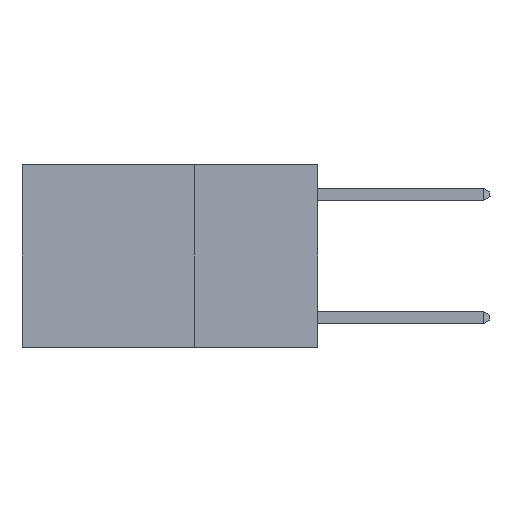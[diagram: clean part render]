
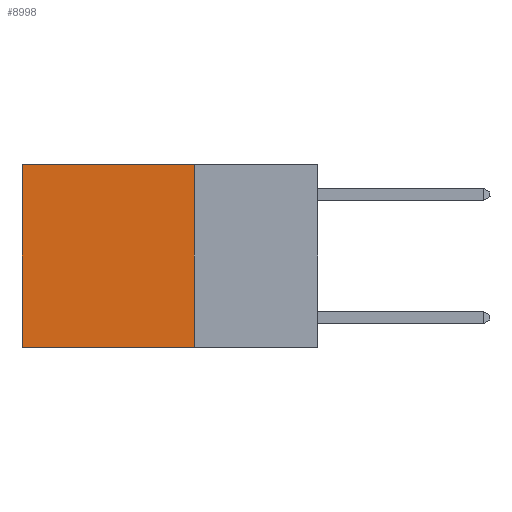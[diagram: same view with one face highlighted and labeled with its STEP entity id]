
A CAD part, left-side view. The second image highlights one B-rep face of the part: STEP entity #8998.
In plain terms, the highlighted planar face has unit normal (-1, 0, 0).
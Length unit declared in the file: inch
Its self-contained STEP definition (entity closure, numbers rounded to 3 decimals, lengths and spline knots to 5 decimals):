
#612 = DIRECTION ( 'NONE',  ( 0., 1., 0. ) ) ;
#2070 = AXIS2_PLACEMENT_3D ( 'NONE', #14344, #12523, #6757 ) ;
#2288 = VERTEX_POINT ( 'NONE', #7746 ) ;
#2604 = CARTESIAN_POINT ( 'NONE',  ( 0.2625, 0.6, -0.37 ) ) ;
#3311 = ORIENTED_EDGE ( 'NONE', *, *, #24102, .F. ) ;
#3319 = EDGE_CURVE ( 'NONE', #2288, #22652, #19076, .T. ) ;
#6757 = DIRECTION ( 'NONE',  ( 0., 0., -1. ) ) ;
#6874 = CARTESIAN_POINT ( 'NONE',  ( 0.2625, 0.25, -0.37 ) ) ;
#7277 = DIRECTION ( 'NONE',  ( 0., 0., -1. ) ) ;
#7364 = LINE ( 'NONE', #8428, #9677 ) ;
#7407 = EDGE_LOOP ( 'NONE', ( #20145, #8150, #3311, #14377 ) ) ;
#7746 = CARTESIAN_POINT ( 'NONE',  ( 0.2625, 0.6, 0. ) ) ;
#8150 = ORIENTED_EDGE ( 'NONE', *, *, #18836, .F. ) ;
#8239 = VECTOR ( 'NONE', #23655, 39.37008 ) ;
#8428 = CARTESIAN_POINT ( 'NONE',  ( 0.2625, 0.25, 0. ) ) ;
#8555 = FACE_OUTER_BOUND ( 'NONE', #7407, .T. ) ;
#8998 = ADVANCED_FACE ( 'NONE', ( #8555 ), #21666, .F. ) ;
#9325 = CARTESIAN_POINT ( 'NONE',  ( 0.2625, 0.25, 0. ) ) ;
#9677 = VECTOR ( 'NONE', #612, 39.37008 ) ;
#10609 = VECTOR ( 'NONE', #7277, 39.37008 ) ;
#11518 = DIRECTION ( 'NONE',  ( 0., 0., -1. ) ) ;
#12523 = DIRECTION ( 'NONE',  ( 1., 0., 0. ) ) ;
#12534 = VERTEX_POINT ( 'NONE', #16650 ) ;
#12620 = VECTOR ( 'NONE', #11518, 39.37008 ) ;
#14344 = CARTESIAN_POINT ( 'NONE',  ( 0.2625, 0.25, 0. ) ) ;
#14377 = ORIENTED_EDGE ( 'NONE', *, *, #19549, .T. ) ;
#14919 = LINE ( 'NONE', #6874, #8239 ) ;
#15792 = CARTESIAN_POINT ( 'NONE',  ( 0.2625, 0.25, 0. ) ) ;
#16650 = CARTESIAN_POINT ( 'NONE',  ( 0.2625, 0.25, -0.37 ) ) ;
#17655 = LINE ( 'NONE', #9325, #10609 ) ;
#18784 = CARTESIAN_POINT ( 'NONE',  ( 0.2625, 0.6, 0. ) ) ;
#18836 = EDGE_CURVE ( 'NONE', #12534, #22652, #14919, .T. ) ;
#19076 = LINE ( 'NONE', #18784, #12620 ) ;
#19266 = VERTEX_POINT ( 'NONE', #15792 ) ;
#19549 = EDGE_CURVE ( 'NONE', #19266, #2288, #7364, .T. ) ;
#20145 = ORIENTED_EDGE ( 'NONE', *, *, #3319, .T. ) ;
#21666 = PLANE ( 'NONE',  #2070 ) ;
#22652 = VERTEX_POINT ( 'NONE', #2604 ) ;
#23655 = DIRECTION ( 'NONE',  ( 0., 1., 0. ) ) ;
#24102 = EDGE_CURVE ( 'NONE', #19266, #12534, #17655, .T. ) ;
